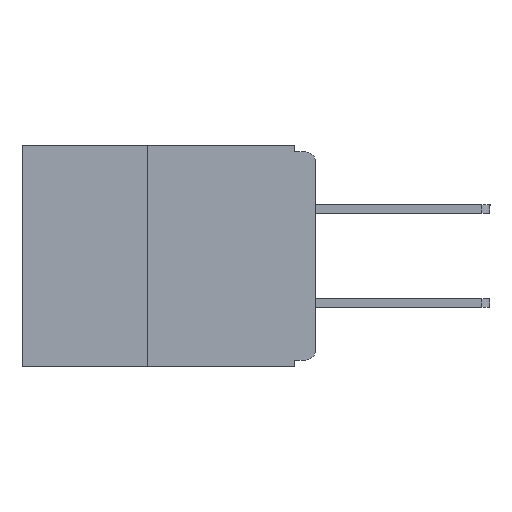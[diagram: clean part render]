
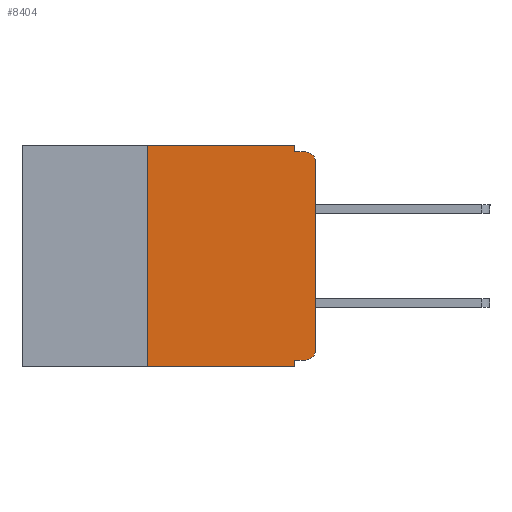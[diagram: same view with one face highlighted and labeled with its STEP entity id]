
A CAD part, left-side view. The second image highlights one B-rep face of the part: STEP entity #8404.
In plain terms, the highlighted planar face has unit normal (-1, 0, 0).
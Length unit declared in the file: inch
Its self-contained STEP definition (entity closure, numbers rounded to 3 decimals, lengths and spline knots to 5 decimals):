
#31 = VERTEX_POINT ( 'NONE', #10076 ) ;
#59 = CARTESIAN_POINT ( 'NONE',  ( 0., 0.25, -0.33 ) ) ;
#220 = PLANE ( 'NONE',  #5779 ) ;
#227 = DIRECTION ( 'NONE',  ( 0., 1., 0. ) ) ;
#589 = CARTESIAN_POINT ( 'NONE',  ( 0., 0.25, 0. ) ) ;
#617 = LINE ( 'NONE', #8457, #11169 ) ;
#657 = CARTESIAN_POINT ( 'NONE',  ( 0., 0., -0.32 ) ) ;
#709 = VERTEX_POINT ( 'NONE', #9645 ) ;
#832 = EDGE_CURVE ( 'NONE', #10094, #11552, #2419, .T. ) ;
#873 = AXIS2_PLACEMENT_3D ( 'NONE', #9588, #9540, #9511 ) ;
#1119 = DIRECTION ( 'NONE',  ( 0., 0., 1. ) ) ;
#1426 = VERTEX_POINT ( 'NONE', #13277 ) ;
#1626 = CARTESIAN_POINT ( 'NONE',  ( 0., 0., -0.01 ) ) ;
#1908 = EDGE_CURVE ( 'NONE', #1426, #31, #10912, .T. ) ;
#2093 = CARTESIAN_POINT ( 'NONE',  ( 0., 0.25, -0.33 ) ) ;
#2248 = DIRECTION ( 'NONE',  ( -1., 0., 0. ) ) ;
#2306 = EDGE_CURVE ( 'NONE', #3313, #11567, #10265, .T. ) ;
#2419 = LINE ( 'NONE', #5948, #10147 ) ;
#2618 = CARTESIAN_POINT ( 'NONE',  ( 0., 0., 0. ) ) ;
#3183 = VERTEX_POINT ( 'NONE', #11205 ) ;
#3232 = EDGE_CURVE ( 'NONE', #1426, #9375, #3318, .T. ) ;
#3235 = DIRECTION ( 'NONE',  ( 0., -1., 0. ) ) ;
#3313 = VERTEX_POINT ( 'NONE', #3986 ) ;
#3318 = LINE ( 'NONE', #657, #6054 ) ;
#3408 = DIRECTION ( 'NONE',  ( 1., 0., 0. ) ) ;
#3464 = ORIENTED_EDGE ( 'NONE', *, *, #832, .T. ) ;
#3568 = VECTOR ( 'NONE', #1119, 39.37008 ) ;
#3650 = DIRECTION ( 'NONE',  ( 0., 0., 1. ) ) ;
#3830 = VECTOR ( 'NONE', #3650, 39.37008 ) ;
#3986 = CARTESIAN_POINT ( 'NONE',  ( 0., 0.031, 0. ) ) ;
#4026 = LINE ( 'NONE', #12167, #9326 ) ;
#4404 = EDGE_LOOP ( 'NONE', ( #10648, #6439, #11506, #10966, #6646, #7079, #3464, #12054, #10098, #6075 ) ) ;
#5607 = CARTESIAN_POINT ( 'NONE',  ( 0., 0.031, -0.01 ) ) ;
#5779 = AXIS2_PLACEMENT_3D ( 'NONE', #8641, #3408, #10765 ) ;
#5948 = CARTESIAN_POINT ( 'NONE',  ( 0., 0.437, -0.33 ) ) ;
#6054 = VECTOR ( 'NONE', #227, 39.37008 ) ;
#6075 = ORIENTED_EDGE ( 'NONE', *, *, #1908, .T. ) ;
#6439 = ORIENTED_EDGE ( 'NONE', *, *, #13126, .T. ) ;
#6646 = ORIENTED_EDGE ( 'NONE', *, *, #8267, .F. ) ;
#6675 = AXIS2_PLACEMENT_3D ( 'NONE', #8522, #2248, #9609 ) ;
#6900 = DIRECTION ( 'NONE',  ( 0., 0., -1. ) ) ;
#7079 = ORIENTED_EDGE ( 'NONE', *, *, #13113, .F. ) ;
#7378 = FACE_OUTER_BOUND ( 'NONE', #4404, .T. ) ;
#8169 = LINE ( 'NONE', #1626, #10366 ) ;
#8267 = EDGE_CURVE ( 'NONE', #11042, #3313, #617, .T. ) ;
#8271 = CARTESIAN_POINT ( 'NONE',  ( 0., 0.031, -0.32 ) ) ;
#8404 = ADVANCED_FACE ( 'NONE', ( #7378 ), #220, .F. ) ;
#8457 = CARTESIAN_POINT ( 'NONE',  ( 0., 0.437, 0. ) ) ;
#8522 = CARTESIAN_POINT ( 'NONE',  ( 0., 0.015, -0.025 ) ) ;
#8641 = CARTESIAN_POINT ( 'NONE',  ( 0., 0.437, 0. ) ) ;
#8857 = CIRCLE ( 'NONE', #6675, 0.015 ) ;
#9326 = VECTOR ( 'NONE', #6900, 39.37008 ) ;
#9375 = VERTEX_POINT ( 'NONE', #8271 ) ;
#9511 = DIRECTION ( 'NONE',  ( 0., 0., -1. ) ) ;
#9532 = LINE ( 'NONE', #59, #3568 ) ;
#9540 = DIRECTION ( 'NONE',  ( -1., 0., 0. ) ) ;
#9588 = CARTESIAN_POINT ( 'NONE',  ( 0., 0.015, -0.305 ) ) ;
#9609 = DIRECTION ( 'NONE',  ( 0., 0., -1. ) ) ;
#9630 = DIRECTION ( 'NONE',  ( 0., 0., -1. ) ) ;
#9645 = CARTESIAN_POINT ( 'NONE',  ( 0., 0., -0.025 ) ) ;
#10061 = DIRECTION ( 'NONE',  ( 0., -1., 0. ) ) ;
#10076 = CARTESIAN_POINT ( 'NONE',  ( 0., 0., -0.305 ) ) ;
#10094 = VERTEX_POINT ( 'NONE', #2093 ) ;
#10098 = ORIENTED_EDGE ( 'NONE', *, *, #3232, .F. ) ;
#10147 = VECTOR ( 'NONE', #12190, 39.37008 ) ;
#10265 = LINE ( 'NONE', #10326, #12680 ) ;
#10326 = CARTESIAN_POINT ( 'NONE',  ( 0., 0.031, 0. ) ) ;
#10366 = VECTOR ( 'NONE', #10061, 39.37008 ) ;
#10477 = EDGE_CURVE ( 'NONE', #9375, #11552, #4026, .T. ) ;
#10648 = ORIENTED_EDGE ( 'NONE', *, *, #12242, .T. ) ;
#10765 = DIRECTION ( 'NONE',  ( 0., 0., -1. ) ) ;
#10912 = CIRCLE ( 'NONE', #873, 0.015 ) ;
#10966 = ORIENTED_EDGE ( 'NONE', *, *, #2306, .F. ) ;
#11042 = VERTEX_POINT ( 'NONE', #589 ) ;
#11169 = VECTOR ( 'NONE', #3235, 39.37008 ) ;
#11205 = CARTESIAN_POINT ( 'NONE',  ( 0., 0.015, -0.01 ) ) ;
#11506 = ORIENTED_EDGE ( 'NONE', *, *, #12787, .F. ) ;
#11552 = VERTEX_POINT ( 'NONE', #12965 ) ;
#11567 = VERTEX_POINT ( 'NONE', #5607 ) ;
#12054 = ORIENTED_EDGE ( 'NONE', *, *, #10477, .F. ) ;
#12167 = CARTESIAN_POINT ( 'NONE',  ( 0., 0.031, -0.33 ) ) ;
#12190 = DIRECTION ( 'NONE',  ( 0., -1., 0. ) ) ;
#12218 = LINE ( 'NONE', #2618, #3830 ) ;
#12242 = EDGE_CURVE ( 'NONE', #31, #709, #12218, .T. ) ;
#12680 = VECTOR ( 'NONE', #9630, 39.37008 ) ;
#12787 = EDGE_CURVE ( 'NONE', #11567, #3183, #8169, .T. ) ;
#12965 = CARTESIAN_POINT ( 'NONE',  ( 0., 0.031, -0.33 ) ) ;
#13113 = EDGE_CURVE ( 'NONE', #10094, #11042, #9532, .T. ) ;
#13126 = EDGE_CURVE ( 'NONE', #709, #3183, #8857, .T. ) ;
#13277 = CARTESIAN_POINT ( 'NONE',  ( 0., 0.015, -0.32 ) ) ;
